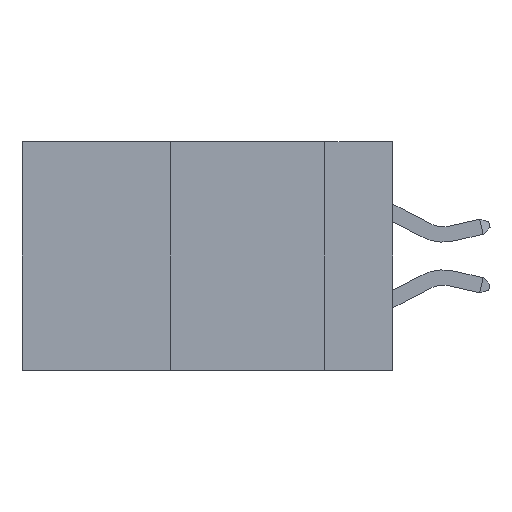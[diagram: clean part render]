
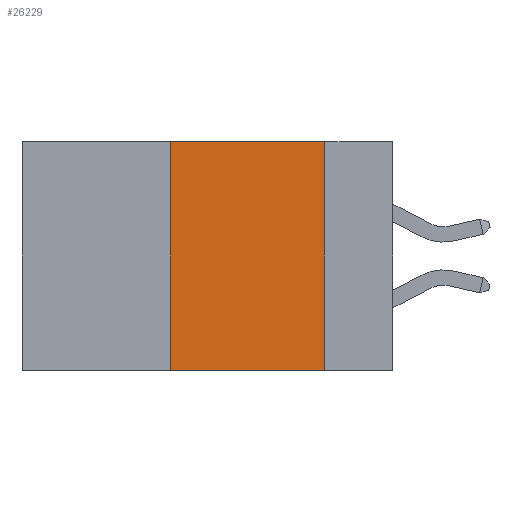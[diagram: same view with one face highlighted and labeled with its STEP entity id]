
A CAD part, left-side view. The second image highlights one B-rep face of the part: STEP entity #26229.
In plain terms, the highlighted planar face has unit normal (-1, 0, 0).
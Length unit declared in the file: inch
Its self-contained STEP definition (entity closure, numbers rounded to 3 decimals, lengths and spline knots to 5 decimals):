
#314 = VECTOR ( 'NONE', #29832, 39.37008 ) ;
#372 = VERTEX_POINT ( 'NONE', #11572 ) ;
#929 = AXIS2_PLACEMENT_3D ( 'NONE', #34665, #14671, #26400 ) ;
#2456 = ORIENTED_EDGE ( 'NONE', *, *, #8300, .F. ) ;
#4366 = LINE ( 'NONE', #6385, #31102 ) ;
#5039 = ORIENTED_EDGE ( 'NONE', *, *, #6075, .T. ) ;
#5270 = VERTEX_POINT ( 'NONE', #32126 ) ;
#6075 = EDGE_CURVE ( 'NONE', #372, #11004, #17917, .T. ) ;
#6385 = CARTESIAN_POINT ( 'NONE',  ( 0., 0.6, 0. ) ) ;
#6875 = DIRECTION ( 'NONE',  ( 0., 0., -1. ) ) ;
#7259 = VECTOR ( 'NONE', #6875, 39.37008 ) ;
#7538 = CARTESIAN_POINT ( 'NONE',  ( 0., 0.11, 0. ) ) ;
#8300 = EDGE_CURVE ( 'NONE', #5270, #13107, #4366, .T. ) ;
#10404 = ORIENTED_EDGE ( 'NONE', *, *, #21513, .F. ) ;
#11004 = VERTEX_POINT ( 'NONE', #33144 ) ;
#11572 = CARTESIAN_POINT ( 'NONE',  ( 0., 0.36, -0.37 ) ) ;
#11833 = EDGE_CURVE ( 'NONE', #372, #5270, #21310, .T. ) ;
#13107 = VERTEX_POINT ( 'NONE', #7538 ) ;
#14671 = DIRECTION ( 'NONE',  ( 1., 0., 0. ) ) ;
#15384 = LINE ( 'NONE', #17593, #7259 ) ;
#17593 = CARTESIAN_POINT ( 'NONE',  ( 0., 0.11, 0. ) ) ;
#17668 = CARTESIAN_POINT ( 'NONE',  ( 0., 0.36, 0. ) ) ;
#17917 = LINE ( 'NONE', #29468, #314 ) ;
#21310 = LINE ( 'NONE', #17668, #28816 ) ;
#21333 = EDGE_LOOP ( 'NONE', ( #10404, #2456, #35850, #5039 ) ) ;
#21513 = EDGE_CURVE ( 'NONE', #13107, #11004, #15384, .T. ) ;
#26229 = ADVANCED_FACE ( 'NONE', ( #31739 ), #31375, .F. ) ;
#26400 = DIRECTION ( 'NONE',  ( 0., 0., -1. ) ) ;
#28816 = VECTOR ( 'NONE', #28847, 39.37008 ) ;
#28832 = DIRECTION ( 'NONE',  ( 0., -1., 0. ) ) ;
#28847 = DIRECTION ( 'NONE',  ( 0., 0., 1. ) ) ;
#29468 = CARTESIAN_POINT ( 'NONE',  ( 0., 0.6, -0.37 ) ) ;
#29832 = DIRECTION ( 'NONE',  ( 0., -1., 0. ) ) ;
#31102 = VECTOR ( 'NONE', #28832, 39.37008 ) ;
#31375 = PLANE ( 'NONE',  #929 ) ;
#31739 = FACE_OUTER_BOUND ( 'NONE', #21333, .T. ) ;
#32126 = CARTESIAN_POINT ( 'NONE',  ( 0., 0.36, 0. ) ) ;
#33144 = CARTESIAN_POINT ( 'NONE',  ( 0., 0.11, -0.37 ) ) ;
#34665 = CARTESIAN_POINT ( 'NONE',  ( 0., 0.6, 0. ) ) ;
#35850 = ORIENTED_EDGE ( 'NONE', *, *, #11833, .F. ) ;
